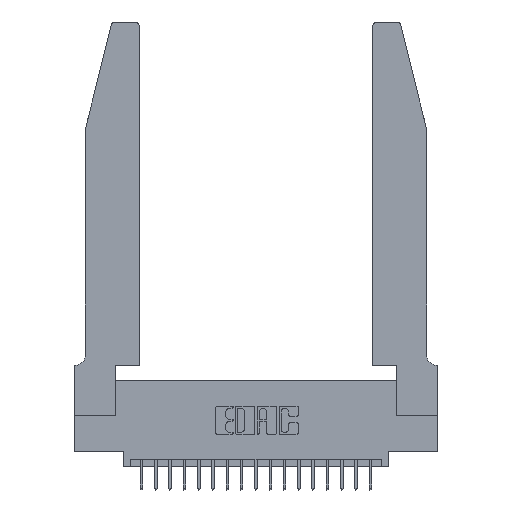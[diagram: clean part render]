
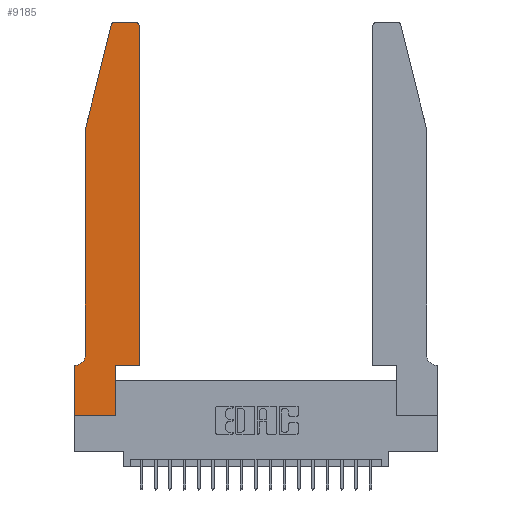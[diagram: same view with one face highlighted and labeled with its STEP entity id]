
A CAD part, top view. The second image highlights one B-rep face of the part: STEP entity #9185.
In plain terms, the highlighted planar face has unit normal (0, 0, 1).
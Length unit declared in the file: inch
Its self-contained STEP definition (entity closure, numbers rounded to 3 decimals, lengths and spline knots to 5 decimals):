
#185 = DIRECTION ( 'NONE',  ( 1., 0., 0. ) ) ;
#552 = CARTESIAN_POINT ( 'NONE',  ( 0.284, 2.72, 0.37 ) ) ;
#637 = DIRECTION ( 'NONE',  ( 1., 0., 0. ) ) ;
#641 = VERTEX_POINT ( 'NONE', #4841 ) ;
#879 = CARTESIAN_POINT ( 'NONE',  ( 0.2865, 0.35, 0.37 ) ) ;
#881 = VERTEX_POINT ( 'NONE', #5135 ) ;
#882 = CARTESIAN_POINT ( 'NONE',  ( 0.0755, 0.42, 0.37 ) ) ;
#950 = EDGE_CURVE ( 'NONE', #6635, #12509, #3141, .T. ) ;
#1141 = DIRECTION ( 'NONE',  ( -1., 0., 0. ) ) ;
#1254 = FACE_OUTER_BOUND ( 'NONE', #5212, .T. ) ;
#1491 = VECTOR ( 'NONE', #18288, 39.37008 ) ;
#1525 = CARTESIAN_POINT ( 'NONE',  ( 0.4505, 2.72, 0.37 ) ) ;
#1857 = ORIENTED_EDGE ( 'NONE', *, *, #9581, .T. ) ;
#1962 = AXIS2_PLACEMENT_3D ( 'NONE', #3975, #3904, #637 ) ;
#2639 = VERTEX_POINT ( 'NONE', #1525 ) ;
#2811 = LINE ( 'NONE', #12369, #15644 ) ;
#2891 = LINE ( 'NONE', #5838, #18077 ) ;
#3091 = LINE ( 'NONE', #11204, #20870 ) ;
#3141 = LINE ( 'NONE', #8443, #18321 ) ;
#3528 = CARTESIAN_POINT ( 'NONE',  ( 0.4505, 0.35, 0.37 ) ) ;
#3904 = DIRECTION ( 'NONE',  ( 0., 0., 1. ) ) ;
#3928 = EDGE_CURVE ( 'NONE', #2639, #15986, #13075, .T. ) ;
#3975 = CARTESIAN_POINT ( 'NONE',  ( 0., 0.35, 0.37 ) ) ;
#4326 = ORIENTED_EDGE ( 'NONE', *, *, #14010, .T. ) ;
#4408 = CARTESIAN_POINT ( 'NONE',  ( 0.0055, 0.35, 0.37 ) ) ;
#4678 = ORIENTED_EDGE ( 'NONE', *, *, #5450, .T. ) ;
#4760 = CARTESIAN_POINT ( 'NONE',  ( 0.2605, 2.75, 0.37 ) ) ;
#4841 = CARTESIAN_POINT ( 'NONE',  ( 0.25487, 2.72718, 0.37 ) ) ;
#5122 = DIRECTION ( 'NONE',  ( 0., 1., 0. ) ) ;
#5135 = CARTESIAN_POINT ( 'NONE',  ( 0., 0., 0.37 ) ) ;
#5212 = EDGE_LOOP ( 'NONE', ( #17759, #11695, #4678, #6380, #14053, #8799, #4326, #18361, #6594, #1857, #10607, #18183 ) ) ;
#5450 = EDGE_CURVE ( 'NONE', #641, #9031, #3091, .T. ) ;
#5616 = DIRECTION ( 'NONE',  ( 1., 0., 0. ) ) ;
#5838 = CARTESIAN_POINT ( 'NONE',  ( 0., 0., 0.37 ) ) ;
#6309 = VERTEX_POINT ( 'NONE', #17902 ) ;
#6380 = ORIENTED_EDGE ( 'NONE', *, *, #9613, .T. ) ;
#6408 = VERTEX_POINT ( 'NONE', #7056 ) ;
#6466 = AXIS2_PLACEMENT_3D ( 'NONE', #8969, #13997, #1141 ) ;
#6594 = ORIENTED_EDGE ( 'NONE', *, *, #9249, .T. ) ;
#6635 = VERTEX_POINT ( 'NONE', #4408 ) ;
#6890 = DIRECTION ( 'NONE',  ( -1., 0., 0. ) ) ;
#7056 = CARTESIAN_POINT ( 'NONE',  ( 0.284, 2.75, 0.37 ) ) ;
#7120 = CARTESIAN_POINT ( 'NONE',  ( 0.2865, 0.35, 0.37 ) ) ;
#7269 = PLANE ( 'NONE',  #1962 ) ;
#8443 = CARTESIAN_POINT ( 'NONE',  ( 0.0755, 0.35, 0.37 ) ) ;
#8799 = ORIENTED_EDGE ( 'NONE', *, *, #950, .T. ) ;
#8969 = CARTESIAN_POINT ( 'NONE',  ( 0.0055, 0.42, 0.37 ) ) ;
#9031 = VERTEX_POINT ( 'NONE', #14945 ) ;
#9185 = ADVANCED_FACE ( 'NONE', ( #1254 ), #7269, .T. ) ;
#9249 = EDGE_CURVE ( 'NONE', #6309, #12008, #12757, .T. ) ;
#9280 = CARTESIAN_POINT ( 'NONE',  ( 0.0755, 2., 0.37 ) ) ;
#9421 = LINE ( 'NONE', #4760, #21440 ) ;
#9462 = DIRECTION ( 'NONE',  ( -0.239, -0.971, 0. ) ) ;
#9486 = EDGE_CURVE ( 'NONE', #6408, #641, #20592, .T. ) ;
#9581 = EDGE_CURVE ( 'NONE', #12008, #16914, #2811, .T. ) ;
#9613 = EDGE_CURVE ( 'NONE', #9031, #14445, #15109, .T. ) ;
#9651 = EDGE_CURVE ( 'NONE', #14445, #6635, #18758, .T. ) ;
#10536 = LINE ( 'NONE', #15294, #13435 ) ;
#10607 = ORIENTED_EDGE ( 'NONE', *, *, #11424, .T. ) ;
#11204 = CARTESIAN_POINT ( 'NONE',  ( 0.0755, 2., 0.37 ) ) ;
#11361 = AXIS2_PLACEMENT_3D ( 'NONE', #552, #17133, #5616 ) ;
#11424 = EDGE_CURVE ( 'NONE', #16914, #2639, #16632, .T. ) ;
#11695 = ORIENTED_EDGE ( 'NONE', *, *, #9486, .T. ) ;
#11736 = CARTESIAN_POINT ( 'NONE',  ( 0.4205, 2.75, 0.37 ) ) ;
#11749 = EDGE_CURVE ( 'NONE', #881, #6309, #10536, .T. ) ;
#12008 = VERTEX_POINT ( 'NONE', #7120 ) ;
#12126 = DIRECTION ( 'NONE',  ( 1., 0., 0. ) ) ;
#12369 = CARTESIAN_POINT ( 'NONE',  ( 0.4505, 0.35, 0.37 ) ) ;
#12509 = VERTEX_POINT ( 'NONE', #19565 ) ;
#12757 = LINE ( 'NONE', #879, #18030 ) ;
#13075 = CIRCLE ( 'NONE', #15392, 0.03 ) ;
#13435 = VECTOR ( 'NONE', #185, 39.37008 ) ;
#13725 = EDGE_CURVE ( 'NONE', #15986, #6408, #9421, .T. ) ;
#13997 = DIRECTION ( 'NONE',  ( 0., 0., -1. ) ) ;
#14010 = EDGE_CURVE ( 'NONE', #12509, #881, #2891, .T. ) ;
#14053 = ORIENTED_EDGE ( 'NONE', *, *, #9651, .T. ) ;
#14445 = VERTEX_POINT ( 'NONE', #882 ) ;
#14638 = CARTESIAN_POINT ( 'NONE',  ( 0.4505, 0.35, 0.37 ) ) ;
#14838 = DIRECTION ( 'NONE',  ( -1., 0., 0. ) ) ;
#14945 = CARTESIAN_POINT ( 'NONE',  ( 0.0755, 2., 0.37 ) ) ;
#15109 = LINE ( 'NONE', #9280, #1491 ) ;
#15294 = CARTESIAN_POINT ( 'NONE',  ( 0., 0., 0.37 ) ) ;
#15392 = AXIS2_PLACEMENT_3D ( 'NONE', #16643, #18585, #12126 ) ;
#15644 = VECTOR ( 'NONE', #18947, 39.37008 ) ;
#15986 = VERTEX_POINT ( 'NONE', #11736 ) ;
#16632 = LINE ( 'NONE', #3528, #21288 ) ;
#16643 = CARTESIAN_POINT ( 'NONE',  ( 0.4205, 2.72, 0.37 ) ) ;
#16914 = VERTEX_POINT ( 'NONE', #14638 ) ;
#17133 = DIRECTION ( 'NONE',  ( 0., 0., 1. ) ) ;
#17759 = ORIENTED_EDGE ( 'NONE', *, *, #13725, .T. ) ;
#17902 = CARTESIAN_POINT ( 'NONE',  ( 0.2865, 0., 0.37 ) ) ;
#18030 = VECTOR ( 'NONE', #21045, 39.37008 ) ;
#18077 = VECTOR ( 'NONE', #19446, 39.37008 ) ;
#18183 = ORIENTED_EDGE ( 'NONE', *, *, #3928, .T. ) ;
#18288 = DIRECTION ( 'NONE',  ( 0., -1., 0. ) ) ;
#18321 = VECTOR ( 'NONE', #6890, 39.37008 ) ;
#18361 = ORIENTED_EDGE ( 'NONE', *, *, #11749, .T. ) ;
#18585 = DIRECTION ( 'NONE',  ( 0., 0., 1. ) ) ;
#18758 = CIRCLE ( 'NONE', #6466, 0.07 ) ;
#18947 = DIRECTION ( 'NONE',  ( 1., 0., 0. ) ) ;
#19446 = DIRECTION ( 'NONE',  ( 0., -1., 0. ) ) ;
#19565 = CARTESIAN_POINT ( 'NONE',  ( 0., 0.35, 0.37 ) ) ;
#20592 = CIRCLE ( 'NONE', #11361, 0.03 ) ;
#20870 = VECTOR ( 'NONE', #9462, 39.37008 ) ;
#21045 = DIRECTION ( 'NONE',  ( 0., 1., 0. ) ) ;
#21288 = VECTOR ( 'NONE', #5122, 39.37008 ) ;
#21440 = VECTOR ( 'NONE', #14838, 39.37008 ) ;
